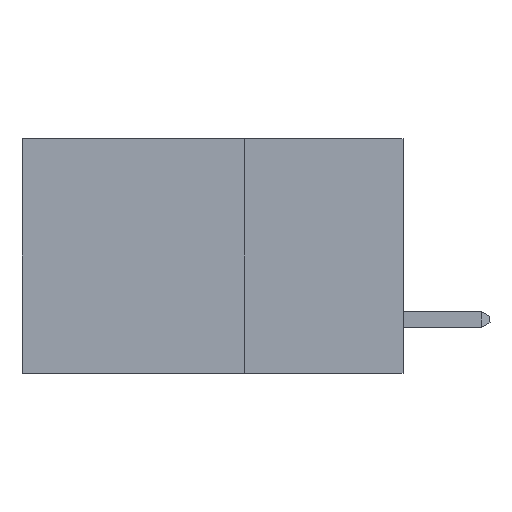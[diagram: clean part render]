
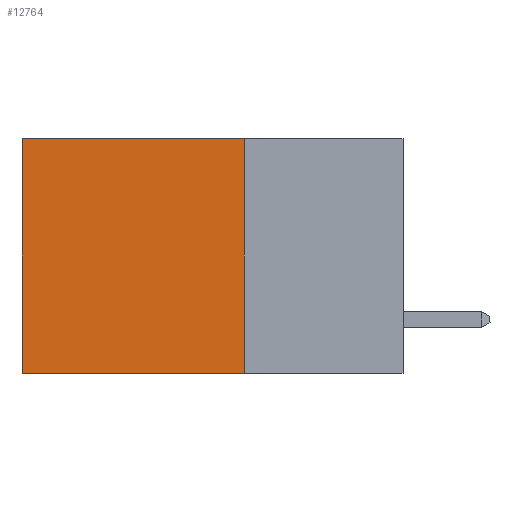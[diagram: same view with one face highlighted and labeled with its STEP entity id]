
A CAD part, left-side view. The second image highlights one B-rep face of the part: STEP entity #12764.
In plain terms, the highlighted planar face has unit normal (-1, 0, 0).
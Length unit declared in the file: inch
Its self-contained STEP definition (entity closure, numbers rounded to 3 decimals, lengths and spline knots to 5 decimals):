
#32 = ORIENTED_EDGE ( 'NONE', *, *, #13645, .F. ) ;
#418 = ORIENTED_EDGE ( 'NONE', *, *, #7695, .T. ) ;
#879 = VECTOR ( 'NONE', #2683, 39.37008 ) ;
#882 = DIRECTION ( 'NONE',  ( 0., 0., -1. ) ) ;
#1521 = CARTESIAN_POINT ( 'NONE',  ( 0.2875, 0.6, 0. ) ) ;
#1842 = VERTEX_POINT ( 'NONE', #3205 ) ;
#2508 = CARTESIAN_POINT ( 'NONE',  ( 0.2875, 0.25, 0. ) ) ;
#2683 = DIRECTION ( 'NONE',  ( 0., 0., -1. ) ) ;
#2834 = PLANE ( 'NONE',  #11820 ) ;
#3179 = CARTESIAN_POINT ( 'NONE',  ( 0.2875, 0.25, -0.37 ) ) ;
#3205 = CARTESIAN_POINT ( 'NONE',  ( 0.2875, 0.6, -0.37 ) ) ;
#3984 = DIRECTION ( 'NONE',  ( 0., 0., -1. ) ) ;
#5528 = VECTOR ( 'NONE', #9388, 39.37008 ) ;
#5604 = LINE ( 'NONE', #11072, #10873 ) ;
#5629 = EDGE_LOOP ( 'NONE', ( #8491, #11697, #32, #418 ) ) ;
#6177 = CARTESIAN_POINT ( 'NONE',  ( 0.2875, 0.6, 0. ) ) ;
#6313 = VERTEX_POINT ( 'NONE', #2508 ) ;
#6514 = VERTEX_POINT ( 'NONE', #6177 ) ;
#6966 = LINE ( 'NONE', #1521, #879 ) ;
#7230 = EDGE_CURVE ( 'NONE', #6514, #1842, #6966, .T. ) ;
#7695 = EDGE_CURVE ( 'NONE', #6313, #6514, #11430, .T. ) ;
#7758 = CARTESIAN_POINT ( 'NONE',  ( 0.2875, 0.25, -0.37 ) ) ;
#8289 = CARTESIAN_POINT ( 'NONE',  ( 0.2875, 0.25, 0. ) ) ;
#8470 = VECTOR ( 'NONE', #14099, 39.37008 ) ;
#8491 = ORIENTED_EDGE ( 'NONE', *, *, #7230, .T. ) ;
#8545 = CARTESIAN_POINT ( 'NONE',  ( 0.2875, 0.25, 0. ) ) ;
#8591 = VERTEX_POINT ( 'NONE', #3179 ) ;
#9388 = DIRECTION ( 'NONE',  ( 0., 1., 0. ) ) ;
#10366 = FACE_OUTER_BOUND ( 'NONE', #5629, .T. ) ;
#10771 = DIRECTION ( 'NONE',  ( 1., 0., 0. ) ) ;
#10873 = VECTOR ( 'NONE', #882, 39.37008 ) ;
#11072 = CARTESIAN_POINT ( 'NONE',  ( 0.2875, 0.25, 0. ) ) ;
#11430 = LINE ( 'NONE', #8289, #5528 ) ;
#11697 = ORIENTED_EDGE ( 'NONE', *, *, #12194, .F. ) ;
#11820 = AXIS2_PLACEMENT_3D ( 'NONE', #8545, #10771, #3984 ) ;
#12003 = LINE ( 'NONE', #7758, #8470 ) ;
#12194 = EDGE_CURVE ( 'NONE', #8591, #1842, #12003, .T. ) ;
#12764 = ADVANCED_FACE ( 'NONE', ( #10366 ), #2834, .F. ) ;
#13645 = EDGE_CURVE ( 'NONE', #6313, #8591, #5604, .T. ) ;
#14099 = DIRECTION ( 'NONE',  ( 0., 1., 0. ) ) ;
